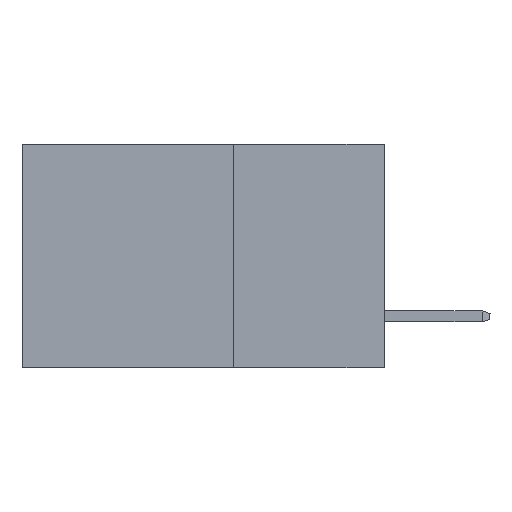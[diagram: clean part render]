
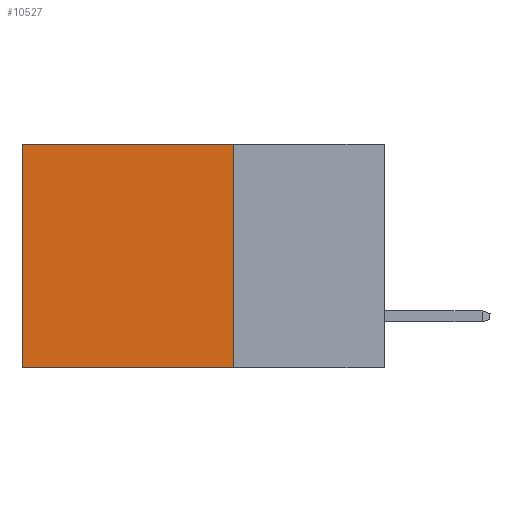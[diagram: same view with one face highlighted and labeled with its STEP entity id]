
A CAD part, left-side view. The second image highlights one B-rep face of the part: STEP entity #10527.
In plain terms, the highlighted planar face has unit normal (-1, 0, 0).
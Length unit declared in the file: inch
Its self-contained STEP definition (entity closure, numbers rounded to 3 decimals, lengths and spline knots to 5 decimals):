
#221 = LINE ( 'NONE', #2160, #11004 ) ;
#302 = DIRECTION ( 'NONE',  ( 0., 1., 0. ) ) ;
#902 = ORIENTED_EDGE ( 'NONE', *, *, #13796, .F. ) ;
#1209 = CARTESIAN_POINT ( 'NONE',  ( 0.2615, 0.25, -0.37 ) ) ;
#1932 = VECTOR ( 'NONE', #302, 39.37008 ) ;
#2160 = CARTESIAN_POINT ( 'NONE',  ( 0.2615, 0.25, -0.37 ) ) ;
#2286 = EDGE_LOOP ( 'NONE', ( #13328, #8717, #902, #6593 ) ) ;
#3676 = CARTESIAN_POINT ( 'NONE',  ( 0.2615, 0.25, -0.37 ) ) ;
#3963 = VECTOR ( 'NONE', #9804, 39.37008 ) ;
#4064 = CARTESIAN_POINT ( 'NONE',  ( 0.2615, 0.6, -0.37 ) ) ;
#6593 = ORIENTED_EDGE ( 'NONE', *, *, #8957, .T. ) ;
#6960 = DIRECTION ( 'NONE',  ( 0., 0., -1. ) ) ;
#7912 = VERTEX_POINT ( 'NONE', #9441 ) ;
#8423 = LINE ( 'NONE', #10823, #1932 ) ;
#8444 = VERTEX_POINT ( 'NONE', #3676 ) ;
#8691 = CARTESIAN_POINT ( 'NONE',  ( 0.2615, 0.25, 0. ) ) ;
#8717 = ORIENTED_EDGE ( 'NONE', *, *, #14890, .F. ) ;
#8957 = EDGE_CURVE ( 'NONE', #9431, #7912, #8423, .T. ) ;
#9431 = VERTEX_POINT ( 'NONE', #8691 ) ;
#9441 = CARTESIAN_POINT ( 'NONE',  ( 0.2615, 0.6, 0. ) ) ;
#9479 = PLANE ( 'NONE',  #11489 ) ;
#9804 = DIRECTION ( 'NONE',  ( 0., 0., -1. ) ) ;
#9824 = LINE ( 'NONE', #4064, #9835 ) ;
#9835 = VECTOR ( 'NONE', #13425, 39.37008 ) ;
#10527 = ADVANCED_FACE ( 'NONE', ( #11800 ), #9479, .F. ) ;
#10737 = CARTESIAN_POINT ( 'NONE',  ( 0.2615, 0.6, -0.37 ) ) ;
#10823 = CARTESIAN_POINT ( 'NONE',  ( 0.2615, 0.25, 0. ) ) ;
#10960 = CARTESIAN_POINT ( 'NONE',  ( 0.2615, 0.25, -0.37 ) ) ;
#11004 = VECTOR ( 'NONE', #13035, 39.37008 ) ;
#11489 = AXIS2_PLACEMENT_3D ( 'NONE', #1209, #13863, #6960 ) ;
#11800 = FACE_OUTER_BOUND ( 'NONE', #2286, .T. ) ;
#12041 = LINE ( 'NONE', #10960, #3963 ) ;
#13035 = DIRECTION ( 'NONE',  ( 0., 1., 0. ) ) ;
#13328 = ORIENTED_EDGE ( 'NONE', *, *, #13368, .T. ) ;
#13368 = EDGE_CURVE ( 'NONE', #7912, #14863, #9824, .T. ) ;
#13425 = DIRECTION ( 'NONE',  ( 0., 0., -1. ) ) ;
#13796 = EDGE_CURVE ( 'NONE', #9431, #8444, #12041, .T. ) ;
#13863 = DIRECTION ( 'NONE',  ( 1., 0., 0. ) ) ;
#14863 = VERTEX_POINT ( 'NONE', #10737 ) ;
#14890 = EDGE_CURVE ( 'NONE', #8444, #14863, #221, .T. ) ;
